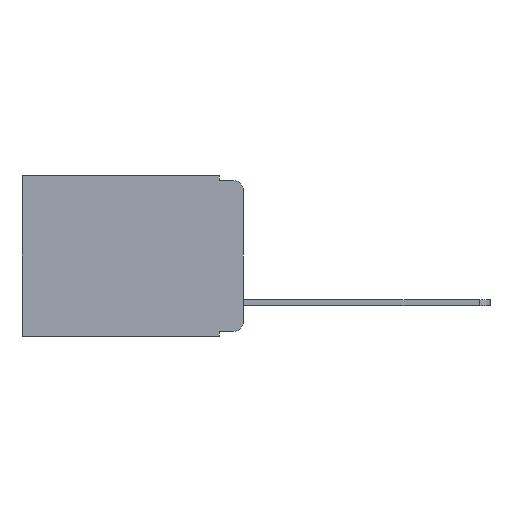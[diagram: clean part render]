
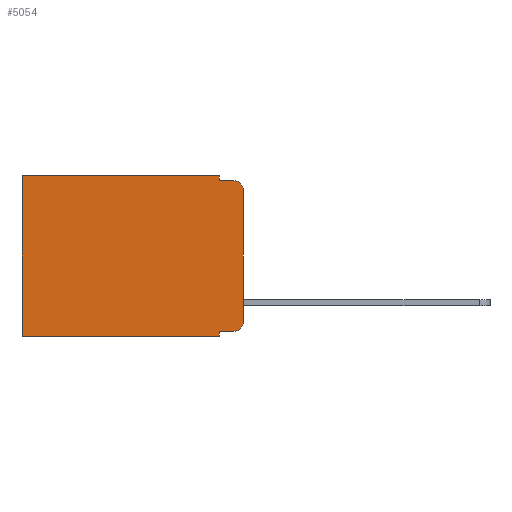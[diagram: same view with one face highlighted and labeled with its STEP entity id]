
A CAD part, left-side view. The second image highlights one B-rep face of the part: STEP entity #5054.
In plain terms, the highlighted planar face has unit normal (-1, 0, 0).
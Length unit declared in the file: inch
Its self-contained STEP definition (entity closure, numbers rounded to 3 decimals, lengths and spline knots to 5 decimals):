
#97 = VERTEX_POINT ( 'NONE', #15908 ) ;
#194 = EDGE_CURVE ( 'NONE', #15730, #17038, #7150, .T. ) ;
#456 = DIRECTION ( 'NONE',  ( 1., 0., 0. ) ) ;
#628 = LINE ( 'NONE', #11909, #13549 ) ;
#634 = CARTESIAN_POINT ( 'NONE',  ( 0.298, 0.473, 0. ) ) ;
#744 = VERTEX_POINT ( 'NONE', #18339 ) ;
#1037 = AXIS2_PLACEMENT_3D ( 'NONE', #1062, #12860, #2814 ) ;
#1062 = CARTESIAN_POINT ( 'NONE',  ( 0.298, 0.02, -0.03 ) ) ;
#1367 = CARTESIAN_POINT ( 'NONE',  ( 0.298, 0.02, -0.313 ) ) ;
#1647 = EDGE_CURVE ( 'NONE', #97, #17038, #1882, .T. ) ;
#1706 = CIRCLE ( 'NONE', #1037, 0.02 ) ;
#1882 = CIRCLE ( 'NONE', #10362, 0.02 ) ;
#1922 = ORIENTED_EDGE ( 'NONE', *, *, #1647, .T. ) ;
#1961 = EDGE_CURVE ( 'NONE', #14704, #2473, #13439, .T. ) ;
#1967 = ORIENTED_EDGE ( 'NONE', *, *, #4423, .F. ) ;
#2473 = VERTEX_POINT ( 'NONE', #7609 ) ;
#2814 = DIRECTION ( 'NONE',  ( 0., 0., -1. ) ) ;
#3261 = VERTEX_POINT ( 'NONE', #634 ) ;
#3656 = CARTESIAN_POINT ( 'NONE',  ( 0.298, 0.051, -0.333 ) ) ;
#4240 = VERTEX_POINT ( 'NONE', #14820 ) ;
#4423 = EDGE_CURVE ( 'NONE', #4240, #19233, #11547, .T. ) ;
#5054 = ADVANCED_FACE ( 'NONE', ( #21377 ), #8933, .F. ) ;
#5353 = DIRECTION ( 'NONE',  ( 0., -1., 0. ) ) ;
#5510 = CARTESIAN_POINT ( 'NONE',  ( 0.298, 0., -0.343 ) ) ;
#5545 = EDGE_CURVE ( 'NONE', #21035, #4240, #628, .T. ) ;
#5649 = CARTESIAN_POINT ( 'NONE',  ( 0.298, 0.473, 0. ) ) ;
#6098 = CARTESIAN_POINT ( 'NONE',  ( 0.298, 0.051, -0.343 ) ) ;
#6238 = LINE ( 'NONE', #19892, #14556 ) ;
#6448 = DIRECTION ( 'NONE',  ( -1., 0., 0. ) ) ;
#7027 = ORIENTED_EDGE ( 'NONE', *, *, #194, .F. ) ;
#7150 = LINE ( 'NONE', #21177, #11605 ) ;
#7363 = DIRECTION ( 'NONE',  ( 0., 0., -1. ) ) ;
#7609 = CARTESIAN_POINT ( 'NONE',  ( 0.298, 0.473, -0.343 ) ) ;
#7777 = VECTOR ( 'NONE', #7363, 39.37008 ) ;
#7850 = CARTESIAN_POINT ( 'NONE',  ( 0.298, 0., 0. ) ) ;
#8013 = EDGE_LOOP ( 'NONE', ( #7027, #20766, #1967, #12751, #13266, #18847, #19353, #20057, #18062, #1922 ) ) ;
#8203 = EDGE_CURVE ( 'NONE', #21035, #3261, #18764, .T. ) ;
#8700 = CARTESIAN_POINT ( 'NONE',  ( 0.298, 0.02, -0.01 ) ) ;
#8933 = PLANE ( 'NONE',  #13579 ) ;
#10362 = AXIS2_PLACEMENT_3D ( 'NONE', #1367, #6448, #19416 ) ;
#10427 = DIRECTION ( 'NONE',  ( 0., -1., 0. ) ) ;
#11547 = LINE ( 'NONE', #16989, #12049 ) ;
#11605 = VECTOR ( 'NONE', #19989, 39.37008 ) ;
#11834 = DIRECTION ( 'NONE',  ( 0., 0., -1. ) ) ;
#11909 = CARTESIAN_POINT ( 'NONE',  ( 0.298, 0.051, 0. ) ) ;
#11910 = CARTESIAN_POINT ( 'NONE',  ( 0.298, 0., -0.03 ) ) ;
#12049 = VECTOR ( 'NONE', #10427, 39.37008 ) ;
#12294 = DIRECTION ( 'NONE',  ( 0., 0., -1. ) ) ;
#12751 = ORIENTED_EDGE ( 'NONE', *, *, #5545, .F. ) ;
#12793 = DIRECTION ( 'NONE',  ( 0., 1., 0. ) ) ;
#12860 = DIRECTION ( 'NONE',  ( -1., 0., 0. ) ) ;
#13266 = ORIENTED_EDGE ( 'NONE', *, *, #8203, .T. ) ;
#13439 = LINE ( 'NONE', #5510, #17232 ) ;
#13549 = VECTOR ( 'NONE', #15166, 39.37008 ) ;
#13579 = AXIS2_PLACEMENT_3D ( 'NONE', #20343, #456, #12294 ) ;
#14275 = VECTOR ( 'NONE', #5353, 39.37008 ) ;
#14491 = VECTOR ( 'NONE', #20905, 39.37008 ) ;
#14556 = VECTOR ( 'NONE', #11834, 39.37008 ) ;
#14704 = VERTEX_POINT ( 'NONE', #6098 ) ;
#14775 = LINE ( 'NONE', #3656, #14275 ) ;
#14820 = CARTESIAN_POINT ( 'NONE',  ( 0.298, 0.051, -0.01 ) ) ;
#15166 = DIRECTION ( 'NONE',  ( 0., 0., -1. ) ) ;
#15320 = EDGE_CURVE ( 'NONE', #15730, #19233, #1706, .T. ) ;
#15329 = CARTESIAN_POINT ( 'NONE',  ( 0.298, 0., -0.313 ) ) ;
#15718 = EDGE_CURVE ( 'NONE', #744, #14704, #6238, .T. ) ;
#15730 = VERTEX_POINT ( 'NONE', #11910 ) ;
#15908 = CARTESIAN_POINT ( 'NONE',  ( 0.298, 0.02, -0.333 ) ) ;
#16406 = EDGE_CURVE ( 'NONE', #744, #97, #14775, .T. ) ;
#16504 = EDGE_CURVE ( 'NONE', #3261, #2473, #20798, .T. ) ;
#16989 = CARTESIAN_POINT ( 'NONE',  ( 0.298, 0.051, -0.01 ) ) ;
#17038 = VERTEX_POINT ( 'NONE', #15329 ) ;
#17232 = VECTOR ( 'NONE', #12793, 39.37008 ) ;
#18062 = ORIENTED_EDGE ( 'NONE', *, *, #16406, .T. ) ;
#18339 = CARTESIAN_POINT ( 'NONE',  ( 0.298, 0.051, -0.333 ) ) ;
#18764 = LINE ( 'NONE', #7850, #14491 ) ;
#18847 = ORIENTED_EDGE ( 'NONE', *, *, #16504, .T. ) ;
#19233 = VERTEX_POINT ( 'NONE', #8700 ) ;
#19353 = ORIENTED_EDGE ( 'NONE', *, *, #1961, .F. ) ;
#19416 = DIRECTION ( 'NONE',  ( 0., 0., -1. ) ) ;
#19892 = CARTESIAN_POINT ( 'NONE',  ( 0.298, 0.051, 0. ) ) ;
#19989 = DIRECTION ( 'NONE',  ( 0., 0., -1. ) ) ;
#20057 = ORIENTED_EDGE ( 'NONE', *, *, #15718, .F. ) ;
#20343 = CARTESIAN_POINT ( 'NONE',  ( 0.298, 0., 0. ) ) ;
#20766 = ORIENTED_EDGE ( 'NONE', *, *, #15320, .T. ) ;
#20798 = LINE ( 'NONE', #5649, #7777 ) ;
#20905 = DIRECTION ( 'NONE',  ( 0., 1., 0. ) ) ;
#21035 = VERTEX_POINT ( 'NONE', #21506 ) ;
#21177 = CARTESIAN_POINT ( 'NONE',  ( 0.298, 0., 0. ) ) ;
#21377 = FACE_OUTER_BOUND ( 'NONE', #8013, .T. ) ;
#21506 = CARTESIAN_POINT ( 'NONE',  ( 0.298, 0.051, 0. ) ) ;
